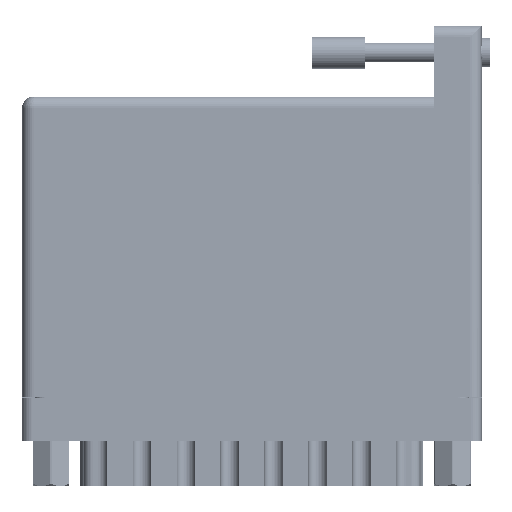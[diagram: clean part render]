
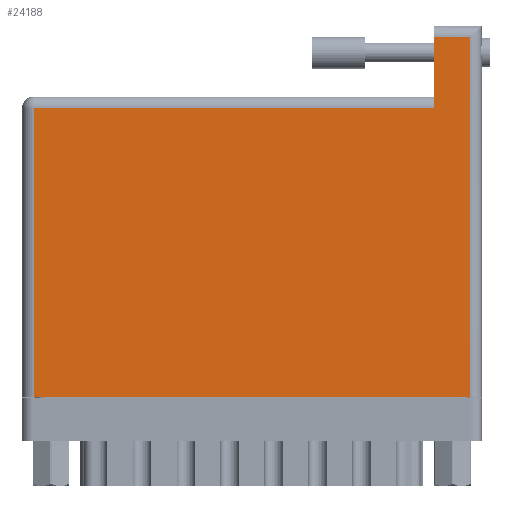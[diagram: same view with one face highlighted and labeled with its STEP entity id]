
A CAD part, front view. The second image highlights one B-rep face of the part: STEP entity #24188.
In plain terms, the highlighted face is planar.
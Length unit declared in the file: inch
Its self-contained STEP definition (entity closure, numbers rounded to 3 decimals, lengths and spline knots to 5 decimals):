
#359 = CARTESIAN_POINT ( 'NONE',  ( 2.648, 0., 0. ) ) ;
#914 = LINE ( 'NONE', #16486, #76690 ) ;
#1746 = VECTOR ( 'NONE', #31679, 39.37008 ) ;
#2039 = CARTESIAN_POINT ( 'NONE',  ( 0., 2.125, 0. ) ) ;
#3454 = CARTESIAN_POINT ( 'NONE',  ( 0., 1.775, 0. ) ) ;
#4063 = EDGE_CURVE ( 'NONE', #85783, #68024, #11944, .T. ) ;
#4339 = VECTOR ( 'NONE', #11353, 39.37008 ) ;
#4993 = CARTESIAN_POINT ( 'NONE',  ( 2.648, 2.195, 0. ) ) ;
#5234 = VECTOR ( 'NONE', #46953, 39.37008 ) ;
#6366 = VERTEX_POINT ( 'NONE', #73188 ) ;
#7318 = FACE_OUTER_BOUND ( 'NONE', #67563, .T. ) ;
#8012 = ORIENTED_EDGE ( 'NONE', *, *, #11437, .T. ) ;
#10309 = DIRECTION ( 'NONE',  ( 0., -1., 0. ) ) ;
#10489 = EDGE_CURVE ( 'NONE', #68024, #61269, #914, .T. ) ;
#11308 = ORIENTED_EDGE ( 'NONE', *, *, #10489, .T. ) ;
#11353 = DIRECTION ( 'NONE',  ( 0., -1., 0. ) ) ;
#11437 = EDGE_CURVE ( 'NONE', #61269, #77988, #58913, .T. ) ;
#11944 = LINE ( 'NONE', #28882, #81553 ) ;
#12174 = CARTESIAN_POINT ( 'NONE',  ( 2.438, 1.705, 0. ) ) ;
#14708 = LINE ( 'NONE', #31660, #4339 ) ;
#16486 = CARTESIAN_POINT ( 'NONE',  ( 0., 0., 0. ) ) ;
#19704 = EDGE_CURVE ( 'NONE', #26557, #85783, #46820, .T. ) ;
#22278 = CARTESIAN_POINT ( 'NONE',  ( 0.07, 1.705, 0. ) ) ;
#24188 = ADVANCED_FACE ( 'NONE', ( #7318 ), #76270, .F. ) ;
#26557 = VERTEX_POINT ( 'NONE', #12174 ) ;
#27055 = ORIENTED_EDGE ( 'NONE', *, *, #28803, .T. ) ;
#28803 = EDGE_CURVE ( 'NONE', #77988, #6366, #33496, .T. ) ;
#28882 = CARTESIAN_POINT ( 'NONE',  ( 0.07, 0., 0. ) ) ;
#31660 = CARTESIAN_POINT ( 'NONE',  ( 2.438, 2.195, 0. ) ) ;
#31679 = DIRECTION ( 'NONE',  ( 0., 1., 0. ) ) ;
#33496 = LINE ( 'NONE', #2039, #49125 ) ;
#37680 = DIRECTION ( 'NONE',  ( 0., 0., -1. ) ) ;
#38212 = AXIS2_PLACEMENT_3D ( 'NONE', #3454, #37680, #43813 ) ;
#39459 = ORIENTED_EDGE ( 'NONE', *, *, #51411, .T. ) ;
#43813 = DIRECTION ( 'NONE',  ( -1., 0., 0. ) ) ;
#44190 = ORIENTED_EDGE ( 'NONE', *, *, #4063, .T. ) ;
#46667 = CARTESIAN_POINT ( 'NONE',  ( 0., 1.705, 0. ) ) ;
#46820 = LINE ( 'NONE', #46667, #5234 ) ;
#46953 = DIRECTION ( 'NONE',  ( -1., 0., 0. ) ) ;
#49125 = VECTOR ( 'NONE', #75464, 39.37008 ) ;
#49905 = DIRECTION ( 'NONE',  ( 1., 0., 0. ) ) ;
#51411 = EDGE_CURVE ( 'NONE', #6366, #26557, #14708, .T. ) ;
#58913 = LINE ( 'NONE', #4993, #1746 ) ;
#61269 = VERTEX_POINT ( 'NONE', #359 ) ;
#63540 = ORIENTED_EDGE ( 'NONE', *, *, #19704, .T. ) ;
#67563 = EDGE_LOOP ( 'NONE', ( #63540, #44190, #11308, #8012, #27055, #39459 ) ) ;
#68024 = VERTEX_POINT ( 'NONE', #79863 ) ;
#73188 = CARTESIAN_POINT ( 'NONE',  ( 2.438, 2.125, 0. ) ) ;
#75464 = DIRECTION ( 'NONE',  ( -1., 0., 0. ) ) ;
#76270 = PLANE ( 'NONE',  #38212 ) ;
#76690 = VECTOR ( 'NONE', #49905, 39.37008 ) ;
#77988 = VERTEX_POINT ( 'NONE', #81252 ) ;
#79863 = CARTESIAN_POINT ( 'NONE',  ( 0.07, 0., 0. ) ) ;
#81252 = CARTESIAN_POINT ( 'NONE',  ( 2.648, 2.125, 0. ) ) ;
#81553 = VECTOR ( 'NONE', #10309, 39.37008 ) ;
#85783 = VERTEX_POINT ( 'NONE', #22278 ) ;
